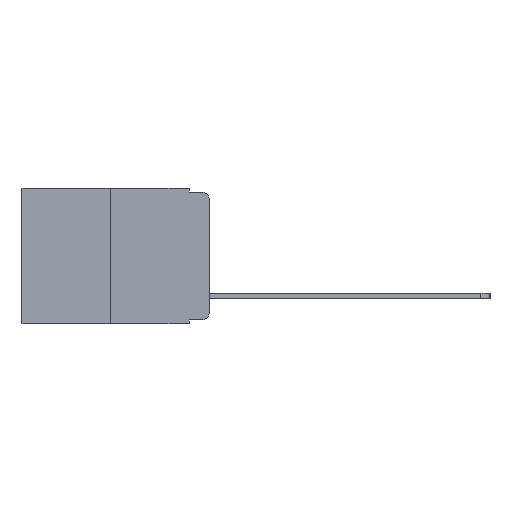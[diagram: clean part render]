
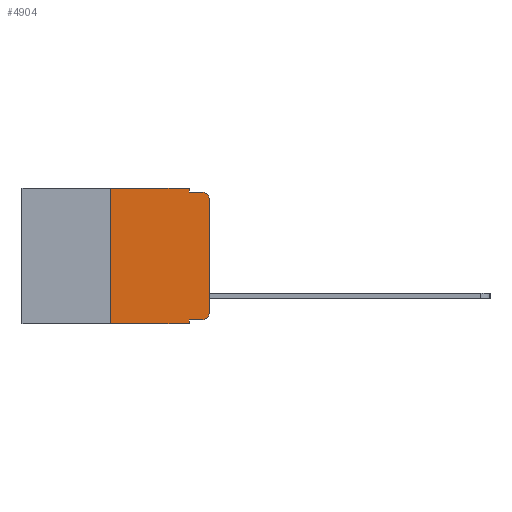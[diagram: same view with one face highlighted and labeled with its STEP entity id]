
A CAD part, left-side view. The second image highlights one B-rep face of the part: STEP entity #4904.
In plain terms, the highlighted planar face has unit normal (-1, 0, 0).
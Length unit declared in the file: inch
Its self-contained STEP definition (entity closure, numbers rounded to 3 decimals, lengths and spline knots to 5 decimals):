
#276 = LINE ( 'NONE', #5735, #3041 ) ;
#584 = VECTOR ( 'NONE', #6597, 39.37008 ) ;
#869 = DIRECTION ( 'NONE',  ( 0., 0., -1. ) ) ;
#1848 = DIRECTION ( 'NONE',  ( 0., 0., -1. ) ) ;
#1916 = CARTESIAN_POINT ( 'NONE',  ( 0., 0.473, 0. ) ) ;
#1946 = VERTEX_POINT ( 'NONE', #8112 ) ;
#2082 = DIRECTION ( 'NONE',  ( 0., -1., 0. ) ) ;
#2083 = VERTEX_POINT ( 'NONE', #7072 ) ;
#2112 = VERTEX_POINT ( 'NONE', #3590 ) ;
#2259 = VECTOR ( 'NONE', #14253, 39.37008 ) ;
#2562 = VERTEX_POINT ( 'NONE', #6818 ) ;
#2675 = VECTOR ( 'NONE', #7700, 39.37008 ) ;
#2716 = CARTESIAN_POINT ( 'NONE',  ( 0., 0., 0. ) ) ;
#2871 = AXIS2_PLACEMENT_3D ( 'NONE', #3454, #11800, #4671 ) ;
#3041 = VECTOR ( 'NONE', #4595, 39.37008 ) ;
#3179 = FACE_OUTER_BOUND ( 'NONE', #3772, .T. ) ;
#3225 = CARTESIAN_POINT ( 'NONE',  ( 0., 0.02, -0.03 ) ) ;
#3454 = CARTESIAN_POINT ( 'NONE',  ( 0., 0.02, -0.313 ) ) ;
#3590 = CARTESIAN_POINT ( 'NONE',  ( 0., 0., -0.03 ) ) ;
#3674 = CIRCLE ( 'NONE', #2871, 0.02 ) ;
#3772 = EDGE_LOOP ( 'NONE', ( #8999, #5493, #3812, #9018, #7242, #7256, #7437, #7609, #9388, #9288 ) ) ;
#3788 = CIRCLE ( 'NONE', #3830, 0.02 ) ;
#3812 = ORIENTED_EDGE ( 'NONE', *, *, #13813, .F. ) ;
#3830 = AXIS2_PLACEMENT_3D ( 'NONE', #3225, #11586, #4433 ) ;
#3943 = VERTEX_POINT ( 'NONE', #10861 ) ;
#4404 = PLANE ( 'NONE',  #4679 ) ;
#4433 = DIRECTION ( 'NONE',  ( 0., 0., -1. ) ) ;
#4534 = CARTESIAN_POINT ( 'NONE',  ( 0., 0.051, 0. ) ) ;
#4595 = DIRECTION ( 'NONE',  ( 0., 0., 1. ) ) ;
#4671 = DIRECTION ( 'NONE',  ( 0., 0., -1. ) ) ;
#4679 = AXIS2_PLACEMENT_3D ( 'NONE', #1916, #5604, #13862 ) ;
#4904 = ADVANCED_FACE ( 'NONE', ( #3179 ), #4404, .F. ) ;
#5493 = ORIENTED_EDGE ( 'NONE', *, *, #14568, .T. ) ;
#5604 = DIRECTION ( 'NONE',  ( 1., 0., 0. ) ) ;
#5636 = LINE ( 'NONE', #2716, #8446 ) ;
#5735 = CARTESIAN_POINT ( 'NONE',  ( 0., 0.25, 0. ) ) ;
#6059 = CARTESIAN_POINT ( 'NONE',  ( 0., 0.473, 0. ) ) ;
#6597 = DIRECTION ( 'NONE',  ( 0., -1., 0. ) ) ;
#6695 = EDGE_CURVE ( 'NONE', #8983, #7882, #3674, .T. ) ;
#6818 = CARTESIAN_POINT ( 'NONE',  ( 0., 0.02, -0.01 ) ) ;
#7072 = CARTESIAN_POINT ( 'NONE',  ( 0., 0.25, 0. ) ) ;
#7242 = ORIENTED_EDGE ( 'NONE', *, *, #9522, .F. ) ;
#7256 = ORIENTED_EDGE ( 'NONE', *, *, #9910, .F. ) ;
#7437 = ORIENTED_EDGE ( 'NONE', *, *, #14003, .T. ) ;
#7558 = LINE ( 'NONE', #14904, #13463 ) ;
#7591 = LINE ( 'NONE', #12514, #584 ) ;
#7609 = ORIENTED_EDGE ( 'NONE', *, *, #9113, .F. ) ;
#7700 = DIRECTION ( 'NONE',  ( 0., -1., 0. ) ) ;
#7882 = VERTEX_POINT ( 'NONE', #10549 ) ;
#8112 = CARTESIAN_POINT ( 'NONE',  ( 0., 0.051, -0.01 ) ) ;
#8306 = EDGE_CURVE ( 'NONE', #3943, #8983, #15246, .T. ) ;
#8446 = VECTOR ( 'NONE', #12269, 39.37008 ) ;
#8856 = VECTOR ( 'NONE', #2082, 39.37008 ) ;
#8908 = CARTESIAN_POINT ( 'NONE',  ( 0., 0.051, -0.333 ) ) ;
#8983 = VERTEX_POINT ( 'NONE', #10053 ) ;
#8999 = ORIENTED_EDGE ( 'NONE', *, *, #15331, .T. ) ;
#9018 = ORIENTED_EDGE ( 'NONE', *, *, #12260, .F. ) ;
#9113 = EDGE_CURVE ( 'NONE', #3943, #15152, #7558, .T. ) ;
#9254 = LINE ( 'NONE', #11694, #8856 ) ;
#9288 = ORIENTED_EDGE ( 'NONE', *, *, #6695, .T. ) ;
#9388 = ORIENTED_EDGE ( 'NONE', *, *, #8306, .T. ) ;
#9457 = CARTESIAN_POINT ( 'NONE',  ( 0., 0.051, -0.343 ) ) ;
#9522 = EDGE_CURVE ( 'NONE', #2083, #12876, #11831, .T. ) ;
#9900 = LINE ( 'NONE', #10664, #15687 ) ;
#9910 = EDGE_CURVE ( 'NONE', #12933, #2083, #276, .T. ) ;
#10053 = CARTESIAN_POINT ( 'NONE',  ( 0., 0.02, -0.333 ) ) ;
#10549 = CARTESIAN_POINT ( 'NONE',  ( 0., 0., -0.313 ) ) ;
#10644 = CARTESIAN_POINT ( 'NONE',  ( 0., 0.25, -0.343 ) ) ;
#10664 = CARTESIAN_POINT ( 'NONE',  ( 0., 0.051, 0. ) ) ;
#10861 = CARTESIAN_POINT ( 'NONE',  ( 0., 0.051, -0.333 ) ) ;
#11586 = DIRECTION ( 'NONE',  ( -1., 0., 0. ) ) ;
#11694 = CARTESIAN_POINT ( 'NONE',  ( 0., 0.473, -0.343 ) ) ;
#11800 = DIRECTION ( 'NONE',  ( -1., 0., 0. ) ) ;
#11831 = LINE ( 'NONE', #6059, #2259 ) ;
#12260 = EDGE_CURVE ( 'NONE', #12876, #1946, #9900, .T. ) ;
#12269 = DIRECTION ( 'NONE',  ( 0., 0., 1. ) ) ;
#12514 = CARTESIAN_POINT ( 'NONE',  ( 0., 0.051, -0.01 ) ) ;
#12876 = VERTEX_POINT ( 'NONE', #4534 ) ;
#12933 = VERTEX_POINT ( 'NONE', #10644 ) ;
#13463 = VECTOR ( 'NONE', #1848, 39.37008 ) ;
#13813 = EDGE_CURVE ( 'NONE', #1946, #2562, #7591, .T. ) ;
#13862 = DIRECTION ( 'NONE',  ( 0., 0., -1. ) ) ;
#14003 = EDGE_CURVE ( 'NONE', #12933, #15152, #9254, .T. ) ;
#14253 = DIRECTION ( 'NONE',  ( 0., -1., 0. ) ) ;
#14568 = EDGE_CURVE ( 'NONE', #2112, #2562, #3788, .T. ) ;
#14904 = CARTESIAN_POINT ( 'NONE',  ( 0., 0.051, 0. ) ) ;
#15152 = VERTEX_POINT ( 'NONE', #9457 ) ;
#15246 = LINE ( 'NONE', #8908, #2675 ) ;
#15331 = EDGE_CURVE ( 'NONE', #7882, #2112, #5636, .T. ) ;
#15687 = VECTOR ( 'NONE', #869, 39.37008 ) ;
